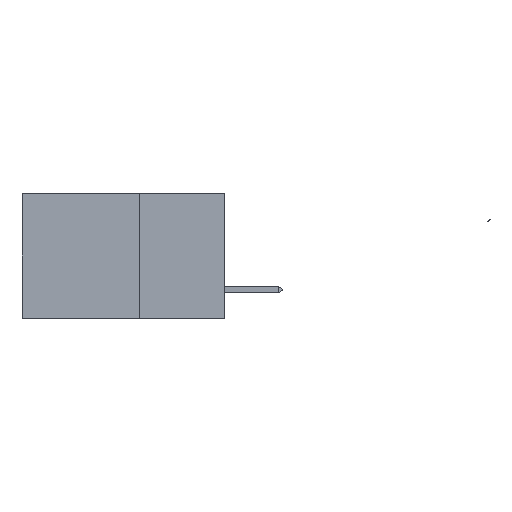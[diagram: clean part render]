
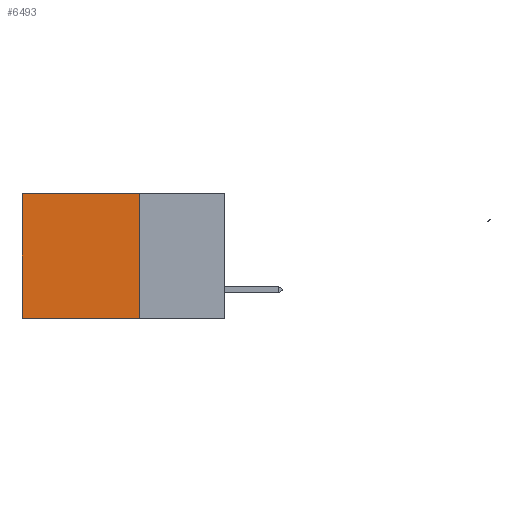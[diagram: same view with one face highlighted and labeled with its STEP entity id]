
A CAD part, left-side view. The second image highlights one B-rep face of the part: STEP entity #6493.
In plain terms, the highlighted planar face has unit normal (-1, 0, 0).
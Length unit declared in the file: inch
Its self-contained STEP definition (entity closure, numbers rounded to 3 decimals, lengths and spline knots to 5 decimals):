
#415 = LINE ( 'NONE', #13761, #10776 ) ;
#447 = LINE ( 'NONE', #10131, #11235 ) ;
#2503 = ORIENTED_EDGE ( 'NONE', *, *, #9005, .T. ) ;
#2507 = EDGE_CURVE ( 'NONE', #16556, #8006, #447, .T. ) ;
#2556 = CARTESIAN_POINT ( 'NONE',  ( 0.2875, 0.6, -0.37 ) ) ;
#2657 = EDGE_CURVE ( 'NONE', #10680, #5157, #5818, .T. ) ;
#3301 = PLANE ( 'NONE',  #14126 ) ;
#3617 = CARTESIAN_POINT ( 'NONE',  ( 0.2875, 0.25, 0. ) ) ;
#4713 = DIRECTION ( 'NONE',  ( 0., 0., -1. ) ) ;
#4775 = EDGE_CURVE ( 'NONE', #5157, #8006, #6159, .T. ) ;
#4882 = CARTESIAN_POINT ( 'NONE',  ( 0.2875, 0.25, 0. ) ) ;
#4984 = ORIENTED_EDGE ( 'NONE', *, *, #2657, .F. ) ;
#5157 = VERTEX_POINT ( 'NONE', #14408 ) ;
#5818 = LINE ( 'NONE', #4882, #13148 ) ;
#6159 = LINE ( 'NONE', #16373, #16735 ) ;
#6311 = DIRECTION ( 'NONE',  ( 0., 0., -1. ) ) ;
#6493 = ADVANCED_FACE ( 'NONE', ( #7216 ), #3301, .F. ) ;
#7216 = FACE_OUTER_BOUND ( 'NONE', #14253, .T. ) ;
#8006 = VERTEX_POINT ( 'NONE', #2556 ) ;
#9005 = EDGE_CURVE ( 'NONE', #10680, #16556, #415, .T. ) ;
#10131 = CARTESIAN_POINT ( 'NONE',  ( 0.2875, 0.6, 0. ) ) ;
#10680 = VERTEX_POINT ( 'NONE', #3617 ) ;
#10776 = VECTOR ( 'NONE', #12436, 39.37008 ) ;
#11235 = VECTOR ( 'NONE', #12825, 39.37008 ) ;
#11636 = ORIENTED_EDGE ( 'NONE', *, *, #2507, .T. ) ;
#12436 = DIRECTION ( 'NONE',  ( 0., 1., 0. ) ) ;
#12825 = DIRECTION ( 'NONE',  ( 0., 0., -1. ) ) ;
#13013 = DIRECTION ( 'NONE',  ( 1., 0., 0. ) ) ;
#13148 = VECTOR ( 'NONE', #6311, 39.37008 ) ;
#13761 = CARTESIAN_POINT ( 'NONE',  ( 0.2875, 0.25, 0. ) ) ;
#14126 = AXIS2_PLACEMENT_3D ( 'NONE', #17137, #13013, #4713 ) ;
#14253 = EDGE_LOOP ( 'NONE', ( #11636, #17366, #4984, #2503 ) ) ;
#14408 = CARTESIAN_POINT ( 'NONE',  ( 0.2875, 0.25, -0.37 ) ) ;
#14992 = DIRECTION ( 'NONE',  ( 0., 1., 0. ) ) ;
#16373 = CARTESIAN_POINT ( 'NONE',  ( 0.2875, 0.25, -0.37 ) ) ;
#16556 = VERTEX_POINT ( 'NONE', #17975 ) ;
#16735 = VECTOR ( 'NONE', #14992, 39.37008 ) ;
#17137 = CARTESIAN_POINT ( 'NONE',  ( 0.2875, 0.25, 0. ) ) ;
#17366 = ORIENTED_EDGE ( 'NONE', *, *, #4775, .F. ) ;
#17975 = CARTESIAN_POINT ( 'NONE',  ( 0.2875, 0.6, 0. ) ) ;
